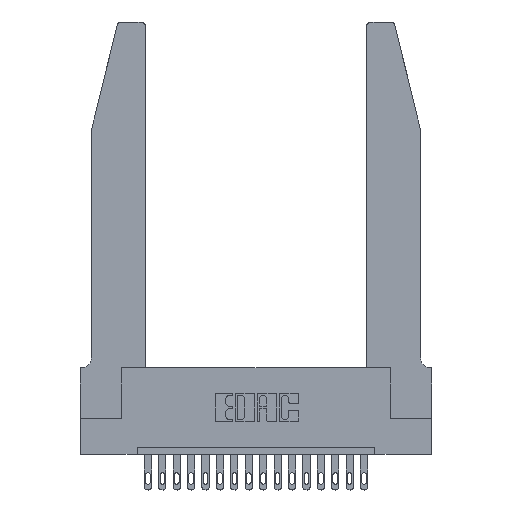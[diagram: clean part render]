
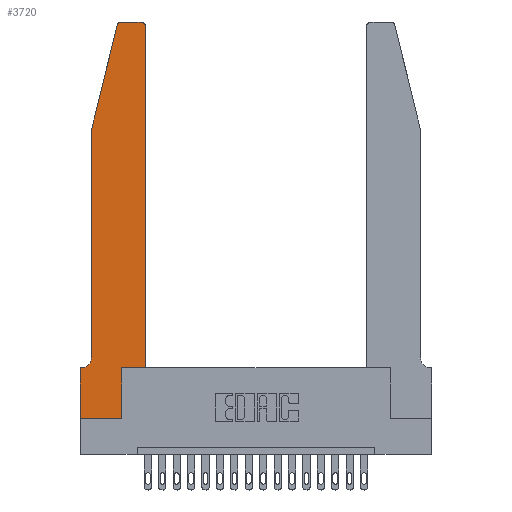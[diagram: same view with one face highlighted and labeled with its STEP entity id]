
A CAD part, top view. The second image highlights one B-rep face of the part: STEP entity #3720.
In plain terms, the highlighted planar face has unit normal (0, 0, 1).
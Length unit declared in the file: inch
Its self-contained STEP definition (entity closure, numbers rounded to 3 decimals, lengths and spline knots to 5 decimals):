
#56 = ORIENTED_EDGE ( 'NONE', *, *, #6876, .T. ) ;
#281 = VERTEX_POINT ( 'NONE', #17628 ) ;
#523 = CARTESIAN_POINT ( 'NONE',  ( 0.0755, 0.35, 0.37 ) ) ;
#576 = VERTEX_POINT ( 'NONE', #15433 ) ;
#641 = DIRECTION ( 'NONE',  ( 0., 0., -1. ) ) ;
#730 = CARTESIAN_POINT ( 'NONE',  ( 0., 0., 0.37 ) ) ;
#881 = DIRECTION ( 'NONE',  ( 1., 0., 0. ) ) ;
#887 = ORIENTED_EDGE ( 'NONE', *, *, #19384, .T. ) ;
#1030 = CIRCLE ( 'NONE', #2904, 0.03 ) ;
#1152 = DIRECTION ( 'NONE',  ( 0., 0., 1. ) ) ;
#1406 = VECTOR ( 'NONE', #9059, 39.37008 ) ;
#1487 = EDGE_CURVE ( 'NONE', #10173, #8461, #16844, .T. ) ;
#2327 = AXIS2_PLACEMENT_3D ( 'NONE', #8460, #641, #9997 ) ;
#2424 = DIRECTION ( 'NONE',  ( 1., 0., 0. ) ) ;
#2689 = CARTESIAN_POINT ( 'NONE',  ( 0., 0.35, 0.37 ) ) ;
#2852 = LINE ( 'NONE', #10457, #1406 ) ;
#2898 = DIRECTION ( 'NONE',  ( 0., 0., 1. ) ) ;
#2904 = AXIS2_PLACEMENT_3D ( 'NONE', #18587, #15962, #12697 ) ;
#3131 = VECTOR ( 'NONE', #881, 39.37008 ) ;
#3257 = DIRECTION ( 'NONE',  ( 0., -1., 0. ) ) ;
#3367 = VECTOR ( 'NONE', #11752, 39.37008 ) ;
#3538 = EDGE_CURVE ( 'NONE', #17157, #16747, #12414, .T. ) ;
#3567 = EDGE_CURVE ( 'NONE', #15452, #18885, #13386, .T. ) ;
#3720 = ADVANCED_FACE ( 'NONE', ( #18001 ), #4082, .T. ) ;
#3954 = CARTESIAN_POINT ( 'NONE',  ( 0.0755, 2., 0.37 ) ) ;
#3975 = VECTOR ( 'NONE', #3257, 39.37008 ) ;
#4082 = PLANE ( 'NONE',  #11032 ) ;
#4205 = CARTESIAN_POINT ( 'NONE',  ( 0.4205, 2.72, 0.37 ) ) ;
#4498 = ORIENTED_EDGE ( 'NONE', *, *, #1487, .T. ) ;
#5172 = EDGE_CURVE ( 'NONE', #16747, #10173, #15735, .T. ) ;
#5204 = EDGE_CURVE ( 'NONE', #18540, #281, #6958, .T. ) ;
#5257 = VERTEX_POINT ( 'NONE', #20153 ) ;
#6000 = ORIENTED_EDGE ( 'NONE', *, *, #13611, .T. ) ;
#6115 = VERTEX_POINT ( 'NONE', #8800 ) ;
#6200 = EDGE_LOOP ( 'NONE', ( #14723, #56, #20173, #887, #8328, #18591, #4498, #13776, #14450, #6000, #17815, #18969 ) ) ;
#6274 = LINE ( 'NONE', #12975, #12897 ) ;
#6679 = VECTOR ( 'NONE', #10389, 39.37008 ) ;
#6876 = EDGE_CURVE ( 'NONE', #5257, #18540, #1030, .T. ) ;
#6958 = LINE ( 'NONE', #3954, #6679 ) ;
#7061 = LINE ( 'NONE', #19455, #3131 ) ;
#7370 = VERTEX_POINT ( 'NONE', #14062 ) ;
#7873 = LINE ( 'NONE', #18251, #12504 ) ;
#8172 = LINE ( 'NONE', #18795, #3975 ) ;
#8328 = ORIENTED_EDGE ( 'NONE', *, *, #3538, .T. ) ;
#8460 = CARTESIAN_POINT ( 'NONE',  ( 0.0055, 0.42, 0.37 ) ) ;
#8461 = VERTEX_POINT ( 'NONE', #11265 ) ;
#8800 = CARTESIAN_POINT ( 'NONE',  ( 0.4205, 2.75, 0.37 ) ) ;
#9059 = DIRECTION ( 'NONE',  ( 0., 1., 0. ) ) ;
#9113 = EDGE_CURVE ( 'NONE', #6115, #5257, #6274, .T. ) ;
#9659 = VECTOR ( 'NONE', #15968, 39.37008 ) ;
#9997 = DIRECTION ( 'NONE',  ( -1., 0., 0. ) ) ;
#10173 = VERTEX_POINT ( 'NONE', #2689 ) ;
#10389 = DIRECTION ( 'NONE',  ( -0.239, -0.971, 0. ) ) ;
#10457 = CARTESIAN_POINT ( 'NONE',  ( 0.2865, 0.35, 0.37 ) ) ;
#11032 = AXIS2_PLACEMENT_3D ( 'NONE', #16716, #1152, #2424 ) ;
#11265 = CARTESIAN_POINT ( 'NONE',  ( 0., 0., 0.37 ) ) ;
#11752 = DIRECTION ( 'NONE',  ( 0., -1., 0. ) ) ;
#12130 = CARTESIAN_POINT ( 'NONE',  ( 0.4505, 0.35, 0.37 ) ) ;
#12414 = CIRCLE ( 'NONE', #2327, 0.07 ) ;
#12504 = VECTOR ( 'NONE', #19787, 39.37008 ) ;
#12697 = DIRECTION ( 'NONE',  ( 1., 0., 0. ) ) ;
#12897 = VECTOR ( 'NONE', #14522, 39.37008 ) ;
#12975 = CARTESIAN_POINT ( 'NONE',  ( 0.2605, 2.75, 0.37 ) ) ;
#13386 = LINE ( 'NONE', #12130, #19475 ) ;
#13608 = AXIS2_PLACEMENT_3D ( 'NONE', #4205, #2898, #19983 ) ;
#13611 = EDGE_CURVE ( 'NONE', #576, #15452, #7873, .T. ) ;
#13644 = CARTESIAN_POINT ( 'NONE',  ( 0.25487, 2.72718, 0.37 ) ) ;
#13776 = ORIENTED_EDGE ( 'NONE', *, *, #16554, .T. ) ;
#14038 = CARTESIAN_POINT ( 'NONE',  ( 0.0055, 0.35, 0.37 ) ) ;
#14062 = CARTESIAN_POINT ( 'NONE',  ( 0.2865, 0., 0.37 ) ) ;
#14450 = ORIENTED_EDGE ( 'NONE', *, *, #17369, .T. ) ;
#14522 = DIRECTION ( 'NONE',  ( -1., 0., 0. ) ) ;
#14723 = ORIENTED_EDGE ( 'NONE', *, *, #9113, .T. ) ;
#14977 = DIRECTION ( 'NONE',  ( 0., 1., 0. ) ) ;
#15433 = CARTESIAN_POINT ( 'NONE',  ( 0.2865, 0.35, 0.37 ) ) ;
#15452 = VERTEX_POINT ( 'NONE', #17803 ) ;
#15735 = LINE ( 'NONE', #523, #9659 ) ;
#15962 = DIRECTION ( 'NONE',  ( 0., 0., 1. ) ) ;
#15968 = DIRECTION ( 'NONE',  ( -1., 0., 0. ) ) ;
#16554 = EDGE_CURVE ( 'NONE', #8461, #7370, #7061, .T. ) ;
#16716 = CARTESIAN_POINT ( 'NONE',  ( 0., 0.35, 0.37 ) ) ;
#16747 = VERTEX_POINT ( 'NONE', #14038 ) ;
#16844 = LINE ( 'NONE', #730, #3367 ) ;
#17157 = VERTEX_POINT ( 'NONE', #17642 ) ;
#17369 = EDGE_CURVE ( 'NONE', #7370, #576, #2852, .T. ) ;
#17628 = CARTESIAN_POINT ( 'NONE',  ( 0.0755, 2., 0.37 ) ) ;
#17642 = CARTESIAN_POINT ( 'NONE',  ( 0.0755, 0.42, 0.37 ) ) ;
#17644 = CARTESIAN_POINT ( 'NONE',  ( 0.4505, 2.72, 0.37 ) ) ;
#17803 = CARTESIAN_POINT ( 'NONE',  ( 0.4505, 0.35, 0.37 ) ) ;
#17815 = ORIENTED_EDGE ( 'NONE', *, *, #3567, .T. ) ;
#18001 = FACE_OUTER_BOUND ( 'NONE', #6200, .T. ) ;
#18034 = EDGE_CURVE ( 'NONE', #18885, #6115, #19441, .T. ) ;
#18251 = CARTESIAN_POINT ( 'NONE',  ( 0.4505, 0.35, 0.37 ) ) ;
#18540 = VERTEX_POINT ( 'NONE', #13644 ) ;
#18587 = CARTESIAN_POINT ( 'NONE',  ( 0.284, 2.72, 0.37 ) ) ;
#18591 = ORIENTED_EDGE ( 'NONE', *, *, #5172, .T. ) ;
#18795 = CARTESIAN_POINT ( 'NONE',  ( 0.0755, 2., 0.37 ) ) ;
#18885 = VERTEX_POINT ( 'NONE', #17644 ) ;
#18969 = ORIENTED_EDGE ( 'NONE', *, *, #18034, .T. ) ;
#19384 = EDGE_CURVE ( 'NONE', #281, #17157, #8172, .T. ) ;
#19441 = CIRCLE ( 'NONE', #13608, 0.03 ) ;
#19455 = CARTESIAN_POINT ( 'NONE',  ( 0., 0., 0.37 ) ) ;
#19475 = VECTOR ( 'NONE', #14977, 39.37008 ) ;
#19787 = DIRECTION ( 'NONE',  ( 1., 0., 0. ) ) ;
#19983 = DIRECTION ( 'NONE',  ( 1., 0., 0. ) ) ;
#20153 = CARTESIAN_POINT ( 'NONE',  ( 0.284, 2.75, 0.37 ) ) ;
#20173 = ORIENTED_EDGE ( 'NONE', *, *, #5204, .T. ) ;
